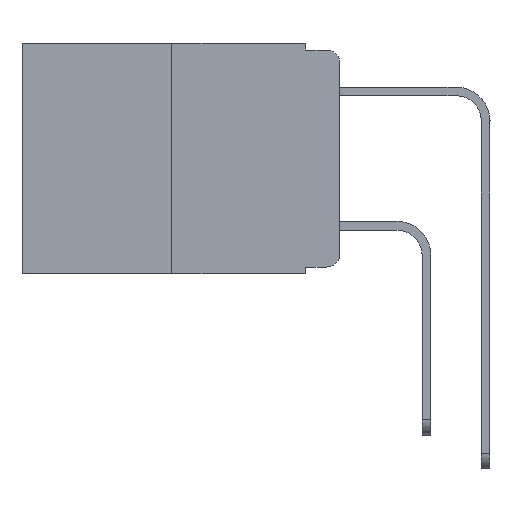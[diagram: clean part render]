
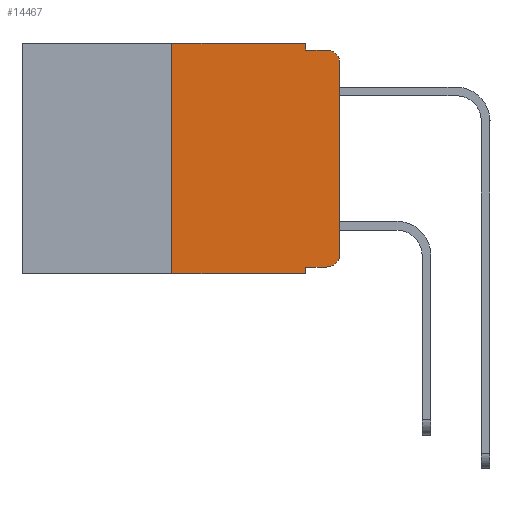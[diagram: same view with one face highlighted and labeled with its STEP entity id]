
A CAD part, left-side view. The second image highlights one B-rep face of the part: STEP entity #14467.
In plain terms, the highlighted planar face has unit normal (-1, 0, 0).
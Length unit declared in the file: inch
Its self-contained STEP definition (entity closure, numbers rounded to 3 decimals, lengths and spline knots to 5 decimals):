
#531 = LINE ( 'NONE', #13812, #15435 ) ;
#747 = LINE ( 'NONE', #2769, #10522 ) ;
#937 = DIRECTION ( 'NONE',  ( 1., 0., 0. ) ) ;
#1249 = EDGE_CURVE ( 'NONE', #11904, #13611, #12396, .T. ) ;
#1715 = AXIS2_PLACEMENT_3D ( 'NONE', #4910, #937, #8823 ) ;
#1756 = EDGE_CURVE ( 'NONE', #22833, #14636, #531, .T. ) ;
#1920 = DIRECTION ( 'NONE',  ( -1., 0., 0. ) ) ;
#1998 = ORIENTED_EDGE ( 'NONE', *, *, #15101, .F. ) ;
#2560 = FACE_OUTER_BOUND ( 'NONE', #4245, .T. ) ;
#2720 = AXIS2_PLACEMENT_3D ( 'NONE', #6196, #19705, #8177 ) ;
#2769 = CARTESIAN_POINT ( 'NONE',  ( 0., 0.051, -0.333 ) ) ;
#3228 = ORIENTED_EDGE ( 'NONE', *, *, #13807, .T. ) ;
#4245 = EDGE_LOOP ( 'NONE', ( #23434, #9324, #24589, #4759, #20763, #11749, #21954, #1998, #22537, #3228 ) ) ;
#4317 = DIRECTION ( 'NONE',  ( 0., 0., 1. ) ) ;
#4759 = ORIENTED_EDGE ( 'NONE', *, *, #21547, .F. ) ;
#4910 = CARTESIAN_POINT ( 'NONE',  ( 0., 0.473, 0. ) ) ;
#5009 = VERTEX_POINT ( 'NONE', #19106 ) ;
#5511 = VERTEX_POINT ( 'NONE', #10240 ) ;
#6196 = CARTESIAN_POINT ( 'NONE',  ( 0., 0.02, -0.313 ) ) ;
#6350 = CARTESIAN_POINT ( 'NONE',  ( 0., 0.473, -0.343 ) ) ;
#6639 = VECTOR ( 'NONE', #11006, 39.37008 ) ;
#6828 = PLANE ( 'NONE',  #1715 ) ;
#7569 = CARTESIAN_POINT ( 'NONE',  ( 0., 0.02, -0.01 ) ) ;
#7642 = CARTESIAN_POINT ( 'NONE',  ( 0., 0.051, 0. ) ) ;
#8177 = DIRECTION ( 'NONE',  ( 0., 0., -1. ) ) ;
#8823 = DIRECTION ( 'NONE',  ( 0., 0., -1. ) ) ;
#8872 = CARTESIAN_POINT ( 'NONE',  ( 0., 0.051, 0. ) ) ;
#9045 = CARTESIAN_POINT ( 'NONE',  ( 0., 0.051, -0.01 ) ) ;
#9324 = ORIENTED_EDGE ( 'NONE', *, *, #21210, .T. ) ;
#9375 = LINE ( 'NONE', #12099, #15106 ) ;
#9397 = CARTESIAN_POINT ( 'NONE',  ( 0., 0., -0.03 ) ) ;
#9588 = CARTESIAN_POINT ( 'NONE',  ( 0., 0.25, -0.343 ) ) ;
#10240 = CARTESIAN_POINT ( 'NONE',  ( 0., 0.02, -0.333 ) ) ;
#10249 = VERTEX_POINT ( 'NONE', #15468 ) ;
#10522 = VECTOR ( 'NONE', #10595, 39.37008 ) ;
#10595 = DIRECTION ( 'NONE',  ( 0., -1., 0. ) ) ;
#10821 = DIRECTION ( 'NONE',  ( 0., 0., -1. ) ) ;
#11006 = DIRECTION ( 'NONE',  ( 0., -1., 0. ) ) ;
#11415 = CIRCLE ( 'NONE', #2720, 0.02 ) ;
#11666 = CARTESIAN_POINT ( 'NONE',  ( 0., 0.473, 0. ) ) ;
#11749 = ORIENTED_EDGE ( 'NONE', *, *, #18931, .F. ) ;
#11904 = VERTEX_POINT ( 'NONE', #12688 ) ;
#12099 = CARTESIAN_POINT ( 'NONE',  ( 0., 0.25, 0. ) ) ;
#12276 = VECTOR ( 'NONE', #10821, 39.37008 ) ;
#12396 = LINE ( 'NONE', #9045, #6639 ) ;
#12555 = EDGE_CURVE ( 'NONE', #17082, #5009, #15408, .T. ) ;
#12688 = CARTESIAN_POINT ( 'NONE',  ( 0., 0.051, -0.01 ) ) ;
#13597 = CARTESIAN_POINT ( 'NONE',  ( 0., 0.02, -0.03 ) ) ;
#13611 = VERTEX_POINT ( 'NONE', #7569 ) ;
#13807 = EDGE_CURVE ( 'NONE', #5511, #22833, #11415, .T. ) ;
#13812 = CARTESIAN_POINT ( 'NONE',  ( 0., 0., 0. ) ) ;
#14362 = VECTOR ( 'NONE', #18656, 39.37008 ) ;
#14467 = ADVANCED_FACE ( 'NONE', ( #2560 ), #6828, .F. ) ;
#14636 = VERTEX_POINT ( 'NONE', #9397 ) ;
#14790 = VECTOR ( 'NONE', #21780, 39.37008 ) ;
#15003 = CARTESIAN_POINT ( 'NONE',  ( 0., 0., -0.313 ) ) ;
#15101 = EDGE_CURVE ( 'NONE', #10249, #5009, #23668, .T. ) ;
#15106 = VECTOR ( 'NONE', #4317, 39.37008 ) ;
#15408 = LINE ( 'NONE', #6350, #14790 ) ;
#15435 = VECTOR ( 'NONE', #22838, 39.37008 ) ;
#15468 = CARTESIAN_POINT ( 'NONE',  ( 0., 0.051, -0.333 ) ) ;
#15507 = DIRECTION ( 'NONE',  ( 0., 0., -1. ) ) ;
#15759 = VERTEX_POINT ( 'NONE', #18417 ) ;
#17051 = CIRCLE ( 'NONE', #17876, 0.02 ) ;
#17082 = VERTEX_POINT ( 'NONE', #9588 ) ;
#17876 = AXIS2_PLACEMENT_3D ( 'NONE', #13597, #1920, #15507 ) ;
#18417 = CARTESIAN_POINT ( 'NONE',  ( 0., 0.25, 0. ) ) ;
#18656 = DIRECTION ( 'NONE',  ( 0., 0., -1. ) ) ;
#18931 = EDGE_CURVE ( 'NONE', #17082, #15759, #9375, .T. ) ;
#19106 = CARTESIAN_POINT ( 'NONE',  ( 0., 0.051, -0.343 ) ) ;
#19431 = EDGE_CURVE ( 'NONE', #15759, #23535, #22872, .T. ) ;
#19705 = DIRECTION ( 'NONE',  ( -1., 0., 0. ) ) ;
#20234 = EDGE_CURVE ( 'NONE', #10249, #5511, #747, .T. ) ;
#20763 = ORIENTED_EDGE ( 'NONE', *, *, #19431, .F. ) ;
#21210 = EDGE_CURVE ( 'NONE', #14636, #13611, #17051, .T. ) ;
#21547 = EDGE_CURVE ( 'NONE', #23535, #11904, #24501, .T. ) ;
#21780 = DIRECTION ( 'NONE',  ( 0., -1., 0. ) ) ;
#21954 = ORIENTED_EDGE ( 'NONE', *, *, #12555, .T. ) ;
#22537 = ORIENTED_EDGE ( 'NONE', *, *, #20234, .T. ) ;
#22601 = CARTESIAN_POINT ( 'NONE',  ( 0., 0.051, 0. ) ) ;
#22833 = VERTEX_POINT ( 'NONE', #15003 ) ;
#22838 = DIRECTION ( 'NONE',  ( 0., 0., 1. ) ) ;
#22872 = LINE ( 'NONE', #11666, #23466 ) ;
#23434 = ORIENTED_EDGE ( 'NONE', *, *, #1756, .T. ) ;
#23466 = VECTOR ( 'NONE', #24947, 39.37008 ) ;
#23535 = VERTEX_POINT ( 'NONE', #7642 ) ;
#23668 = LINE ( 'NONE', #8872, #12276 ) ;
#24501 = LINE ( 'NONE', #22601, #14362 ) ;
#24589 = ORIENTED_EDGE ( 'NONE', *, *, #1249, .F. ) ;
#24947 = DIRECTION ( 'NONE',  ( 0., -1., 0. ) ) ;
